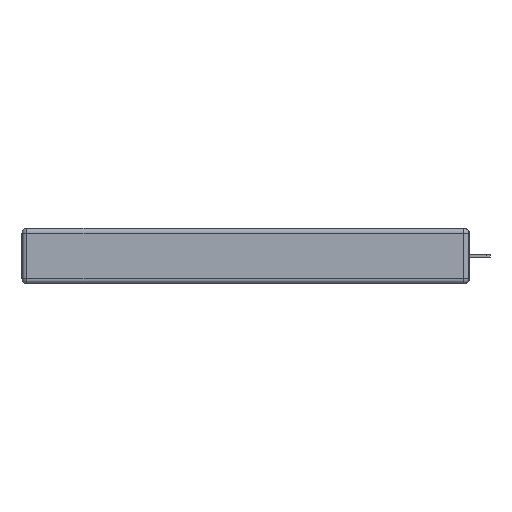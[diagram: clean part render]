
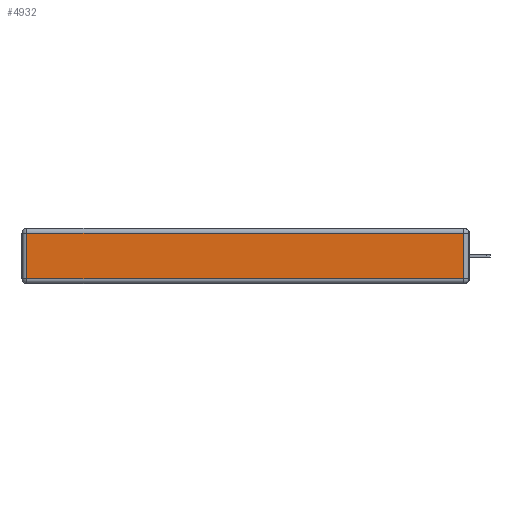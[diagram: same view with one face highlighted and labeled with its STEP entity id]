
A CAD part, left-side view. The second image highlights one B-rep face of the part: STEP entity #4932.
In plain terms, the highlighted planar face has unit normal (-1, 0, 0).
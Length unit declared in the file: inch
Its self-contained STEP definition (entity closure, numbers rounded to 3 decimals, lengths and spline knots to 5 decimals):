
#1720 = CARTESIAN_POINT ( 'NONE',  ( 0., 0.03, -0.313 ) ) ;
#2187 = CARTESIAN_POINT ( 'NONE',  ( 0., 2.72, -0.313 ) ) ;
#2523 = FACE_OUTER_BOUND ( 'NONE', #3406, .T. ) ;
#2715 = ORIENTED_EDGE ( 'NONE', *, *, #24125, .T. ) ;
#3406 = EDGE_LOOP ( 'NONE', ( #11258, #2715, #9312, #18669 ) ) ;
#3439 = VECTOR ( 'NONE', #22301, 39.37008 ) ;
#4001 = LINE ( 'NONE', #13144, #3439 ) ;
#4420 = VECTOR ( 'NONE', #5286, 39.37008 ) ;
#4932 = ADVANCED_FACE ( 'NONE', ( #2523 ), #5364, .T. ) ;
#5286 = DIRECTION ( 'NONE',  ( 0., 1., 0. ) ) ;
#5364 = PLANE ( 'NONE',  #10703 ) ;
#6148 = DIRECTION ( 'NONE',  ( 0., -1., 0. ) ) ;
#6798 = VERTEX_POINT ( 'NONE', #15862 ) ;
#8576 = LINE ( 'NONE', #23537, #12996 ) ;
#9312 = ORIENTED_EDGE ( 'NONE', *, *, #12235, .T. ) ;
#10469 = VERTEX_POINT ( 'NONE', #1720 ) ;
#10703 = AXIS2_PLACEMENT_3D ( 'NONE', #14605, #12392, #12140 ) ;
#11258 = ORIENTED_EDGE ( 'NONE', *, *, #19132, .T. ) ;
#12140 = DIRECTION ( 'NONE',  ( 0., 0., 1. ) ) ;
#12235 = EDGE_CURVE ( 'NONE', #13183, #6798, #20001, .T. ) ;
#12266 = CARTESIAN_POINT ( 'NONE',  ( 0., 0.03, -0.03 ) ) ;
#12392 = DIRECTION ( 'NONE',  ( -1., 0., 0. ) ) ;
#12996 = VECTOR ( 'NONE', #14439, 39.37008 ) ;
#13144 = CARTESIAN_POINT ( 'NONE',  ( 0., 2.72, -0.343 ) ) ;
#13183 = VERTEX_POINT ( 'NONE', #12266 ) ;
#13477 = EDGE_CURVE ( 'NONE', #6798, #17323, #4001, .T. ) ;
#14439 = DIRECTION ( 'NONE',  ( 0., 0., 1. ) ) ;
#14605 = CARTESIAN_POINT ( 'NONE',  ( 0., 0., -0.343 ) ) ;
#15862 = CARTESIAN_POINT ( 'NONE',  ( 0., 2.72, -0.03 ) ) ;
#17323 = VERTEX_POINT ( 'NONE', #2187 ) ;
#18669 = ORIENTED_EDGE ( 'NONE', *, *, #13477, .T. ) ;
#19029 = LINE ( 'NONE', #19255, #24159 ) ;
#19132 = EDGE_CURVE ( 'NONE', #17323, #10469, #19029, .T. ) ;
#19255 = CARTESIAN_POINT ( 'NONE',  ( 0., 0., -0.313 ) ) ;
#20001 = LINE ( 'NONE', #23905, #4420 ) ;
#22301 = DIRECTION ( 'NONE',  ( 0., 0., -1. ) ) ;
#23537 = CARTESIAN_POINT ( 'NONE',  ( 0., 0.03, -0.343 ) ) ;
#23905 = CARTESIAN_POINT ( 'NONE',  ( 0., 2.75, -0.03 ) ) ;
#24125 = EDGE_CURVE ( 'NONE', #10469, #13183, #8576, .T. ) ;
#24159 = VECTOR ( 'NONE', #6148, 39.37008 ) ;
